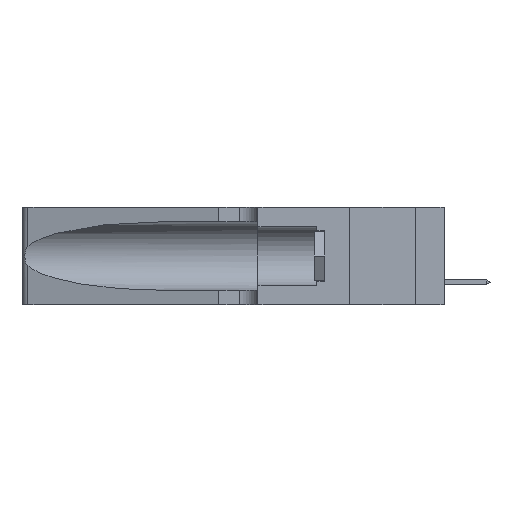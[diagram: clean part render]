
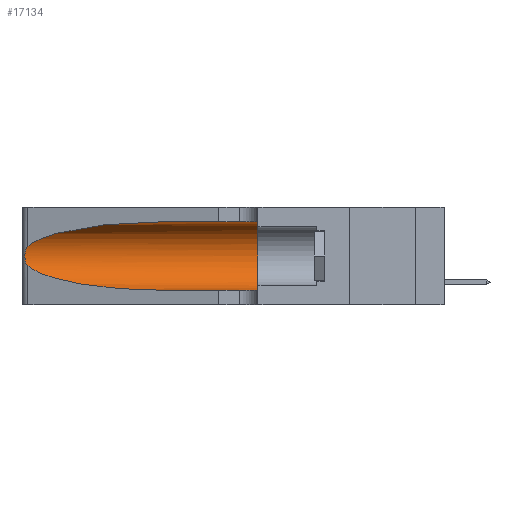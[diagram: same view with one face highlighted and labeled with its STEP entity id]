
A CAD part, left-side view. The second image highlights one B-rep face of the part: STEP entity #17134.
In plain terms, the highlighted cylindrical face has radius 3.308 mm (diameter 6.617 mm), a partial arc.
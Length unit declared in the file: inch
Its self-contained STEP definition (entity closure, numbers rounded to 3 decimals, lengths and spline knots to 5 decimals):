
#605 = CARTESIAN_POINT ( 'NONE',  ( 0.1305, 0.72297, 0.05475 ) ) ;
#921 = CARTESIAN_POINT ( 'NONE',  ( 0.25487, 1.22718, 0.22369 ) ) ;
#935 = VERTEX_POINT ( 'NONE', #5211 ) ;
#1063 = CARTESIAN_POINT ( 'NONE',  ( 0.1305, 1.61858, 0.31525 ) ) ;
#1202 = ORIENTED_EDGE ( 'NONE', *, *, #9014, .T. ) ;
#1900 = DIRECTION ( 'NONE',  ( 0., -1., 0. ) ) ;
#1980 = DIRECTION ( 'NONE',  ( 0., 0., -1. ) ) ;
#2027 = CARTESIAN_POINT ( 'NONE',  ( 0.1305, 0.35, 0.05475 ) ) ;
#2109 = CARTESIAN_POINT ( 'NONE',  ( 0.18966, 0.96281, 0.31525 ) ) ;
#2594 = VERTEX_POINT ( 'NONE', #12409 ) ;
#3318 = ORIENTED_EDGE ( 'NONE', *, *, #7328, .T. ) ;
#3338 =( BOUNDED_CURVE ( )  B_SPLINE_CURVE ( 3, ( #14631, #4048, #13277, #6400 ),
 .UNSPECIFIED., .F., .F. ) 
 B_SPLINE_CURVE_WITH_KNOTS ( ( 4, 4 ),
 ( 3.44316, 4.71239 ),
 .UNSPECIFIED. ) 
 CURVE ( )  GEOMETRIC_REPRESENTATION_ITEM ( )  RATIONAL_B_SPLINE_CURVE ( ( 1., 0.87, 0.87, 1. ) ) 
 REPRESENTATION_ITEM ( '' )  );
#3736 = CARTESIAN_POINT ( 'NONE',  ( 0.25487, 1.22718, 0.22369 ) ) ;
#4048 = CARTESIAN_POINT ( 'NONE',  ( 0.2373, 1.15595, 0.08982 ) ) ;
#4384 = CARTESIAN_POINT ( 'NONE',  ( 0.25789, 1.23486, 0.15765 ) ) ;
#5211 = CARTESIAN_POINT ( 'NONE',  ( 0.25487, 1.22718, 0.14631 ) ) ;
#5512 = EDGE_CURVE ( 'NONE', #15831, #7774, #5545, .T. ) ;
#5545 = CIRCLE ( 'NONE', #21638, 0.13025 ) ;
#5590 = VECTOR ( 'NONE', #8234, 39.37008 ) ;
#6186 = CARTESIAN_POINT ( 'NONE',  ( 0.25555, 1.22993, 0.14849 ) ) ;
#6400 = CARTESIAN_POINT ( 'NONE',  ( 0.1305, 0.72297, 0.05475 ) ) ;
#7055 = CYLINDRICAL_SURFACE ( 'NONE', #21005, 0.13025 ) ;
#7100 = VECTOR ( 'NONE', #21973, 39.37008 ) ;
#7268 = DIRECTION ( 'NONE',  ( 0., 1., 0. ) ) ;
#7328 = EDGE_CURVE ( 'NONE', #935, #17768, #3338, .T. ) ;
#7332 = EDGE_CURVE ( 'NONE', #17768, #7774, #11474, .T. ) ;
#7525 = LINE ( 'NONE', #1063, #5590 ) ;
#7639 = CARTESIAN_POINT ( 'NONE',  ( 0.25639, 1.23184, 0.21858 ) ) ;
#7774 = VERTEX_POINT ( 'NONE', #2027 ) ;
#7853 = CARTESIAN_POINT ( 'NONE',  ( 0.25854, 1.2359, 0.20912 ) ) ;
#8234 = DIRECTION ( 'NONE',  ( 0., -1., 0. ) ) ;
#9014 = EDGE_CURVE ( 'NONE', #2594, #935, #16373, .T. ) ;
#9407 = CARTESIAN_POINT ( 'NONE',  ( 0.26017, 1.23833, 0.17102 ) ) ;
#9560 = CARTESIAN_POINT ( 'NONE',  ( 0.25639, 1.23186, 0.15144 ) ) ;
#10972 = ORIENTED_EDGE ( 'NONE', *, *, #22887, .F. ) ;
#11170 = CARTESIAN_POINT ( 'NONE',  ( 0.25856, 1.23593, 0.16098 ) ) ;
#11474 = LINE ( 'NONE', #18756, #7100 ) ;
#12409 = CARTESIAN_POINT ( 'NONE',  ( 0.25487, 1.22718, 0.22369 ) ) ;
#12469 = CARTESIAN_POINT ( 'NONE',  ( 0.1305, 0.35, 0.185 ) ) ;
#12631 = DIRECTION ( 'NONE',  ( 0., 0., 1. ) ) ;
#12928 = CARTESIAN_POINT ( 'NONE',  ( 0.25487, 1.22718, 0.14631 ) ) ;
#13277 = CARTESIAN_POINT ( 'NONE',  ( 0.18966, 0.96281, 0.05475 ) ) ;
#13738 = CARTESIAN_POINT ( 'NONE',  ( 0.1305, 0.35, 0.31525 ) ) ;
#14474 = CARTESIAN_POINT ( 'NONE',  ( 0.2373, 1.15595, 0.28018 ) ) ;
#14631 = CARTESIAN_POINT ( 'NONE',  ( 0.25487, 1.22718, 0.14631 ) ) ;
#14659 = ORIENTED_EDGE ( 'NONE', *, *, #7332, .T. ) ;
#14893 = CARTESIAN_POINT ( 'NONE',  ( 0.26018, 1.23835, 0.19895 ) ) ;
#14977 = CARTESIAN_POINT ( 'NONE',  ( 0.26075, 1.23896, 0.178 ) ) ;
#15549 = EDGE_LOOP ( 'NONE', ( #22489, #1202, #3318, #14659, #20580, #10972 ) ) ;
#15815 = CARTESIAN_POINT ( 'NONE',  ( 0.1305, 1.61858, 0.185 ) ) ;
#15831 = VERTEX_POINT ( 'NONE', #13738 ) ;
#15868 = CARTESIAN_POINT ( 'NONE',  ( 0.1305, 0.72297, 0.31525 ) ) ;
#16251 = CARTESIAN_POINT ( 'NONE',  ( 0.1305, 0.72297, 0.31525 ) ) ;
#16373 = B_SPLINE_CURVE_WITH_KNOTS ( 'NONE', 3,
 ( #921, #18255, #7639, #21765, #7853, #14893, #16602, #14977, #9407, #11170, #4384, #9560, #6186, #12928 ),
 .UNSPECIFIED., .F., .F.,
 ( 4, 2, 2, 2, 2, 2, 4 ),
 ( 0., 0.00027, 0.00053, 0.00107, 0.0016, 0.00187, 0.00214 ),
 .UNSPECIFIED. ) ;
#16602 = CARTESIAN_POINT ( 'NONE',  ( 0.26075, 1.23896, 0.19203 ) ) ;
#17134 = ADVANCED_FACE ( 'NONE', ( #21975 ), #7055, .F. ) ;
#17768 = VERTEX_POINT ( 'NONE', #605 ) ;
#18130 = VERTEX_POINT ( 'NONE', #15868 ) ;
#18255 = CARTESIAN_POINT ( 'NONE',  ( 0.25555, 1.22994, 0.2215 ) ) ;
#18756 = CARTESIAN_POINT ( 'NONE',  ( 0.1305, 1.61858, 0.05475 ) ) ;
#20364 = EDGE_CURVE ( 'NONE', #18130, #2594, #21178, .T. ) ;
#20580 = ORIENTED_EDGE ( 'NONE', *, *, #5512, .F. ) ;
#21005 = AXIS2_PLACEMENT_3D ( 'NONE', #15815, #1900, #1980 ) ;
#21178 =( BOUNDED_CURVE ( )  B_SPLINE_CURVE ( 3, ( #16251, #2109, #14474, #3736 ),
 .UNSPECIFIED., .F., .T. ) 
 B_SPLINE_CURVE_WITH_KNOTS ( ( 4, 4 ),
 ( 1.5708, 2.84003 ),
 .UNSPECIFIED. ) 
 CURVE ( )  GEOMETRIC_REPRESENTATION_ITEM ( )  RATIONAL_B_SPLINE_CURVE ( ( 1., 0.87, 0.87, 1. ) ) 
 REPRESENTATION_ITEM ( '' )  );
#21638 = AXIS2_PLACEMENT_3D ( 'NONE', #12469, #7268, #12631 ) ;
#21765 = CARTESIAN_POINT ( 'NONE',  ( 0.25787, 1.23484, 0.2124 ) ) ;
#21973 = DIRECTION ( 'NONE',  ( 0., -1., 0. ) ) ;
#21975 = FACE_OUTER_BOUND ( 'NONE', #15549, .T. ) ;
#22489 = ORIENTED_EDGE ( 'NONE', *, *, #20364, .T. ) ;
#22887 = EDGE_CURVE ( 'NONE', #18130, #15831, #7525, .T. ) ;
